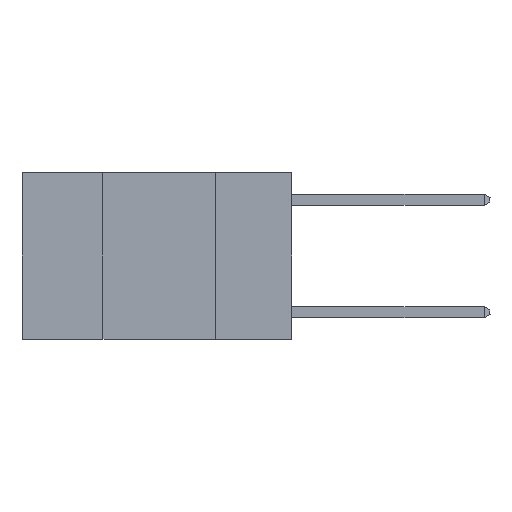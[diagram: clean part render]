
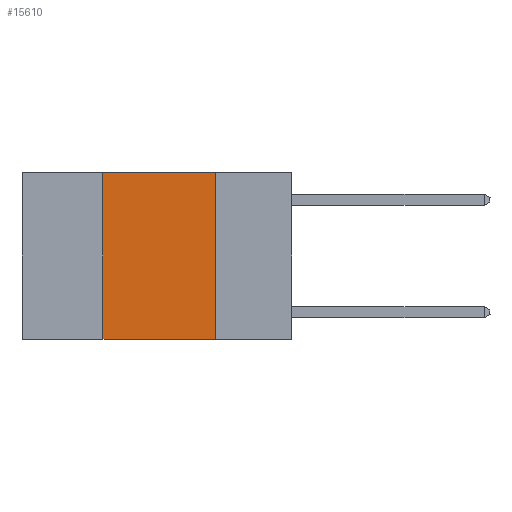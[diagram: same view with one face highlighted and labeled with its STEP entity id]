
A CAD part, left-side view. The second image highlights one B-rep face of the part: STEP entity #15610.
In plain terms, the highlighted planar face has unit normal (-1, 0, 0).
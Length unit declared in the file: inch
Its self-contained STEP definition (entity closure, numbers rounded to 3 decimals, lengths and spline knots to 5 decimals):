
#405 = ORIENTED_EDGE ( 'NONE', *, *, #16802, .F. ) ;
#532 = LINE ( 'NONE', #19614, #13111 ) ;
#964 = DIRECTION ( 'NONE',  ( 0., -1., 0. ) ) ;
#1031 = FACE_OUTER_BOUND ( 'NONE', #21461, .T. ) ;
#1276 = PLANE ( 'NONE',  #4174 ) ;
#1594 = CARTESIAN_POINT ( 'NONE',  ( 0., 0.17, -0.37 ) ) ;
#1688 = VECTOR ( 'NONE', #9718, 39.37008 ) ;
#3867 = ORIENTED_EDGE ( 'NONE', *, *, #14171, .F. ) ;
#4174 = AXIS2_PLACEMENT_3D ( 'NONE', #8656, #19158, #4476 ) ;
#4316 = CARTESIAN_POINT ( 'NONE',  ( 0., 0.6, -0.37 ) ) ;
#4476 = DIRECTION ( 'NONE',  ( 0., 0., -1. ) ) ;
#5008 = CARTESIAN_POINT ( 'NONE',  ( 0., 0.42, -0.37 ) ) ;
#5406 = VERTEX_POINT ( 'NONE', #5008 ) ;
#5599 = CARTESIAN_POINT ( 'NONE',  ( 0., 0.17, 0. ) ) ;
#8423 = EDGE_CURVE ( 'NONE', #5406, #13916, #15272, .T. ) ;
#8656 = CARTESIAN_POINT ( 'NONE',  ( 0., 0.6, 0. ) ) ;
#9278 = VECTOR ( 'NONE', #20952, 39.37008 ) ;
#9718 = DIRECTION ( 'NONE',  ( 0., -1., 0. ) ) ;
#9916 = LINE ( 'NONE', #21153, #20660 ) ;
#11015 = EDGE_CURVE ( 'NONE', #22779, #13916, #532, .T. ) ;
#11105 = VERTEX_POINT ( 'NONE', #19832 ) ;
#13111 = VECTOR ( 'NONE', #23350, 39.37008 ) ;
#13916 = VERTEX_POINT ( 'NONE', #1594 ) ;
#14171 = EDGE_CURVE ( 'NONE', #11105, #22779, #9916, .T. ) ;
#15272 = LINE ( 'NONE', #4316, #1688 ) ;
#15610 = ADVANCED_FACE ( 'NONE', ( #1031 ), #1276, .F. ) ;
#15718 = ORIENTED_EDGE ( 'NONE', *, *, #11015, .F. ) ;
#16405 = LINE ( 'NONE', #18813, #9278 ) ;
#16802 = EDGE_CURVE ( 'NONE', #5406, #11105, #16405, .T. ) ;
#18230 = ORIENTED_EDGE ( 'NONE', *, *, #8423, .T. ) ;
#18813 = CARTESIAN_POINT ( 'NONE',  ( 0., 0.42, 0. ) ) ;
#19158 = DIRECTION ( 'NONE',  ( 1., 0., 0. ) ) ;
#19614 = CARTESIAN_POINT ( 'NONE',  ( 0., 0.17, 0. ) ) ;
#19832 = CARTESIAN_POINT ( 'NONE',  ( 0., 0.42, 0. ) ) ;
#20660 = VECTOR ( 'NONE', #964, 39.37008 ) ;
#20952 = DIRECTION ( 'NONE',  ( 0., 0., 1. ) ) ;
#21153 = CARTESIAN_POINT ( 'NONE',  ( 0., 0.6, 0. ) ) ;
#21461 = EDGE_LOOP ( 'NONE', ( #15718, #3867, #405, #18230 ) ) ;
#22779 = VERTEX_POINT ( 'NONE', #5599 ) ;
#23350 = DIRECTION ( 'NONE',  ( 0., 0., -1. ) ) ;
